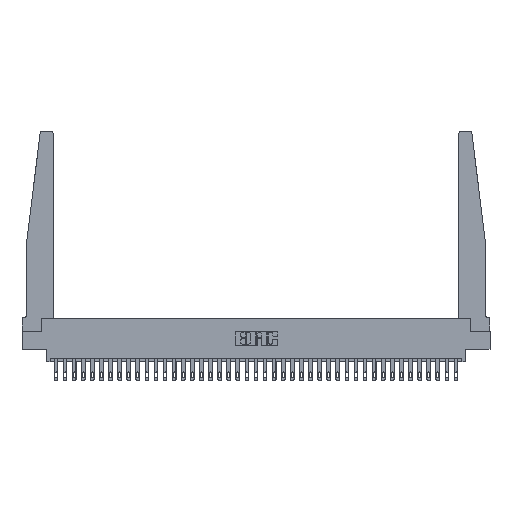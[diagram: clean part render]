
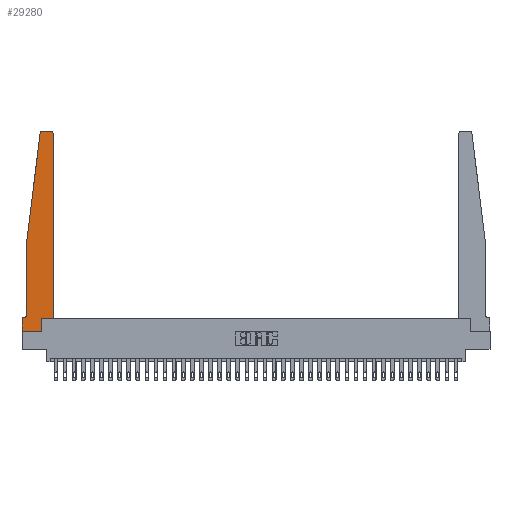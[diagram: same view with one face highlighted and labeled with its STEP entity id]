
A CAD part, top view. The second image highlights one B-rep face of the part: STEP entity #29280.
In plain terms, the highlighted planar face has unit normal (0, 0, 1).
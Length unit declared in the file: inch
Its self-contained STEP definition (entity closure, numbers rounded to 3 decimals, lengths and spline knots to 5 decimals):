
#140 = CARTESIAN_POINT ( 'NONE',  ( 0.065, 0.2375, 0.37 ) ) ;
#682 = VERTEX_POINT ( 'NONE', #4446 ) ;
#965 = DIRECTION ( 'NONE',  ( 1., 0., 0. ) ) ;
#1001 = CARTESIAN_POINT ( 'NONE',  ( 0., 0., 0.37 ) ) ;
#1064 = CARTESIAN_POINT ( 'NONE',  ( 0., 0., 0.37 ) ) ;
#1507 = ORIENTED_EDGE ( 'NONE', *, *, #4181, .T. ) ;
#1536 = DIRECTION ( 'NONE',  ( 1., 0., 0. ) ) ;
#1637 = DIRECTION ( 'NONE',  ( 0., 0., 1. ) ) ;
#1663 = CARTESIAN_POINT ( 'NONE',  ( 0.2605, 0.18, 0.37 ) ) ;
#2005 = VERTEX_POINT ( 'NONE', #33232 ) ;
#2118 = CARTESIAN_POINT ( 'NONE',  ( 0.015, 0.1875, 0.37 ) ) ;
#2627 = EDGE_CURVE ( 'NONE', #12544, #34082, #12555, .T. ) ;
#3904 = CARTESIAN_POINT ( 'NONE',  ( 0.065, 1.25, 0.37 ) ) ;
#3984 = VERTEX_POINT ( 'NONE', #2118 ) ;
#4181 = EDGE_CURVE ( 'NONE', #22937, #9204, #18574, .T. ) ;
#4446 = CARTESIAN_POINT ( 'NONE',  ( 0.27653, 2.75, 0.37 ) ) ;
#4624 = EDGE_CURVE ( 'NONE', #2005, #4910, #19367, .T. ) ;
#4791 = CARTESIAN_POINT ( 'NONE',  ( 0.065, 0.1875, 0.37 ) ) ;
#4910 = VERTEX_POINT ( 'NONE', #15837 ) ;
#5544 = EDGE_CURVE ( 'NONE', #19463, #3984, #23636, .T. ) ;
#6289 = CARTESIAN_POINT ( 'NONE',  ( 0.425, 0.18, 0.37 ) ) ;
#6673 = VECTOR ( 'NONE', #30600, 39.37008 ) ;
#6873 = DIRECTION ( 'NONE',  ( 0., 1., 0. ) ) ;
#6893 = VECTOR ( 'NONE', #14990, 39.37008 ) ;
#6925 = EDGE_CURVE ( 'NONE', #27742, #22937, #19466, .T. ) ;
#8082 = AXIS2_PLACEMENT_3D ( 'NONE', #32747, #24956, #1536 ) ;
#8209 = LINE ( 'NONE', #18770, #14966 ) ;
#8453 = LINE ( 'NONE', #15884, #9970 ) ;
#8514 = CARTESIAN_POINT ( 'NONE',  ( 0.27653, 2.72, 0.37 ) ) ;
#8943 = LINE ( 'NONE', #3904, #6673 ) ;
#9123 = ORIENTED_EDGE ( 'NONE', *, *, #4624, .T. ) ;
#9204 = VERTEX_POINT ( 'NONE', #23696 ) ;
#9399 = CARTESIAN_POINT ( 'NONE',  ( 0.425, 2.72, 0.37 ) ) ;
#9446 = ORIENTED_EDGE ( 'NONE', *, *, #27446, .T. ) ;
#9490 = EDGE_CURVE ( 'NONE', #9204, #682, #8453, .T. ) ;
#9727 = VECTOR ( 'NONE', #26576, 39.37008 ) ;
#9970 = VECTOR ( 'NONE', #26462, 39.37008 ) ;
#10599 = VECTOR ( 'NONE', #16937, 39.37008 ) ;
#10702 = ORIENTED_EDGE ( 'NONE', *, *, #29036, .T. ) ;
#10809 = EDGE_CURVE ( 'NONE', #34082, #2005, #30800, .T. ) ;
#11169 = EDGE_CURVE ( 'NONE', #16861, #31189, #8943, .T. ) ;
#11307 = DIRECTION ( 'NONE',  ( 0., 1., 0. ) ) ;
#11757 = ORIENTED_EDGE ( 'NONE', *, *, #11169, .T. ) ;
#11920 = ORIENTED_EDGE ( 'NONE', *, *, #5544, .T. ) ;
#12544 = VERTEX_POINT ( 'NONE', #27005 ) ;
#12555 = LINE ( 'NONE', #29182, #9727 ) ;
#13080 = EDGE_LOOP ( 'NONE', ( #15353, #17927, #11757, #9446, #11920, #10702, #18718, #25816, #9123, #31471, #32833, #1507 ) ) ;
#13497 = EDGE_CURVE ( 'NONE', #682, #16861, #26668, .T. ) ;
#14966 = VECTOR ( 'NONE', #26389, 39.37008 ) ;
#14990 = DIRECTION ( 'NONE',  ( 1., 0., 0. ) ) ;
#15191 = DIRECTION ( 'NONE',  ( -1., 0., 0. ) ) ;
#15353 = ORIENTED_EDGE ( 'NONE', *, *, #9490, .T. ) ;
#15824 = VECTOR ( 'NONE', #6873, 39.37008 ) ;
#15837 = CARTESIAN_POINT ( 'NONE',  ( 0.2605, 0.18, 0.37 ) ) ;
#15884 = CARTESIAN_POINT ( 'NONE',  ( 0.25, 2.75, 0.37 ) ) ;
#16861 = VERTEX_POINT ( 'NONE', #22106 ) ;
#16937 = DIRECTION ( 'NONE',  ( 1., 0., 0. ) ) ;
#17075 = FACE_OUTER_BOUND ( 'NONE', #13080, .T. ) ;
#17180 = CARTESIAN_POINT ( 'NONE',  ( 0.015, 0.2375, 0.37 ) ) ;
#17408 = LINE ( 'NONE', #25230, #6893 ) ;
#17707 = CARTESIAN_POINT ( 'NONE',  ( 0.425, 0.18, 0.37 ) ) ;
#17927 = ORIENTED_EDGE ( 'NONE', *, *, #13497, .T. ) ;
#18195 = EDGE_CURVE ( 'NONE', #4910, #27742, #17408, .T. ) ;
#18574 = CIRCLE ( 'NONE', #8082, 0.03 ) ;
#18718 = ORIENTED_EDGE ( 'NONE', *, *, #2627, .T. ) ;
#18770 = CARTESIAN_POINT ( 'NONE',  ( 0.065, 1.25, 0.37 ) ) ;
#19367 = LINE ( 'NONE', #1663, #15824 ) ;
#19463 = VERTEX_POINT ( 'NONE', #140 ) ;
#19466 = LINE ( 'NONE', #6289, #30354 ) ;
#21050 = VECTOR ( 'NONE', #15191, 39.37008 ) ;
#22106 = CARTESIAN_POINT ( 'NONE',  ( 0.24675, 2.72367, 0.37 ) ) ;
#22107 = PLANE ( 'NONE',  #22247 ) ;
#22211 = DIRECTION ( 'NONE',  ( 0., 0., -1. ) ) ;
#22247 = AXIS2_PLACEMENT_3D ( 'NONE', #24892, #1637, #965 ) ;
#22937 = VERTEX_POINT ( 'NONE', #9399 ) ;
#23636 = CIRCLE ( 'NONE', #24766, 0.05 ) ;
#23696 = CARTESIAN_POINT ( 'NONE',  ( 0.395, 2.75, 0.37 ) ) ;
#23897 = AXIS2_PLACEMENT_3D ( 'NONE', #8514, #29659, #29137 ) ;
#24766 = AXIS2_PLACEMENT_3D ( 'NONE', #17180, #22211, #30364 ) ;
#24892 = CARTESIAN_POINT ( 'NONE',  ( 0., 0.1875, 0.37 ) ) ;
#24956 = DIRECTION ( 'NONE',  ( 0., 0., 1. ) ) ;
#25230 = CARTESIAN_POINT ( 'NONE',  ( 0.425, 0.18, 0.37 ) ) ;
#25610 = LINE ( 'NONE', #4791, #21050 ) ;
#25816 = ORIENTED_EDGE ( 'NONE', *, *, #10809, .T. ) ;
#26389 = DIRECTION ( 'NONE',  ( 0., -1., 0. ) ) ;
#26462 = DIRECTION ( 'NONE',  ( -1., 0., 0. ) ) ;
#26576 = DIRECTION ( 'NONE',  ( 0., -1., 0. ) ) ;
#26668 = CIRCLE ( 'NONE', #23897, 0.03 ) ;
#27005 = CARTESIAN_POINT ( 'NONE',  ( 0., 0.1875, 0.37 ) ) ;
#27446 = EDGE_CURVE ( 'NONE', #31189, #19463, #8209, .T. ) ;
#27579 = CARTESIAN_POINT ( 'NONE',  ( 0.065, 1.25, 0.37 ) ) ;
#27742 = VERTEX_POINT ( 'NONE', #17707 ) ;
#29036 = EDGE_CURVE ( 'NONE', #3984, #12544, #25610, .T. ) ;
#29137 = DIRECTION ( 'NONE',  ( 1., 0., 0. ) ) ;
#29182 = CARTESIAN_POINT ( 'NONE',  ( 0., 0., 0.37 ) ) ;
#29280 = ADVANCED_FACE ( 'NONE', ( #17075 ), #22107, .T. ) ;
#29659 = DIRECTION ( 'NONE',  ( 0., 0., 1. ) ) ;
#30354 = VECTOR ( 'NONE', #11307, 39.37008 ) ;
#30364 = DIRECTION ( 'NONE',  ( -1., 0., 0. ) ) ;
#30600 = DIRECTION ( 'NONE',  ( -0.122, -0.992, 0. ) ) ;
#30800 = LINE ( 'NONE', #1001, #10599 ) ;
#31189 = VERTEX_POINT ( 'NONE', #27579 ) ;
#31471 = ORIENTED_EDGE ( 'NONE', *, *, #18195, .T. ) ;
#32747 = CARTESIAN_POINT ( 'NONE',  ( 0.395, 2.72, 0.37 ) ) ;
#32833 = ORIENTED_EDGE ( 'NONE', *, *, #6925, .T. ) ;
#33232 = CARTESIAN_POINT ( 'NONE',  ( 0.2605, 0., 0.37 ) ) ;
#34082 = VERTEX_POINT ( 'NONE', #1064 ) ;
